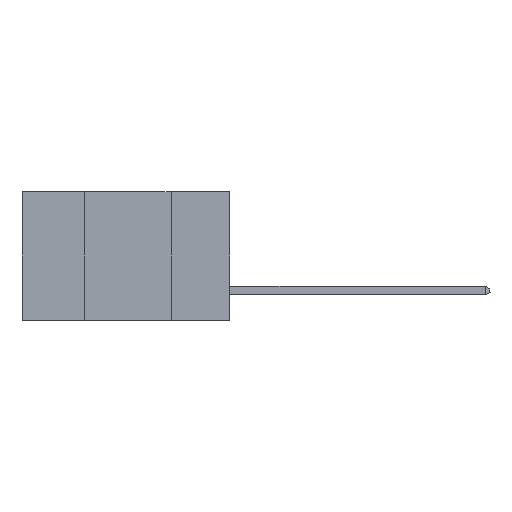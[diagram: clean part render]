
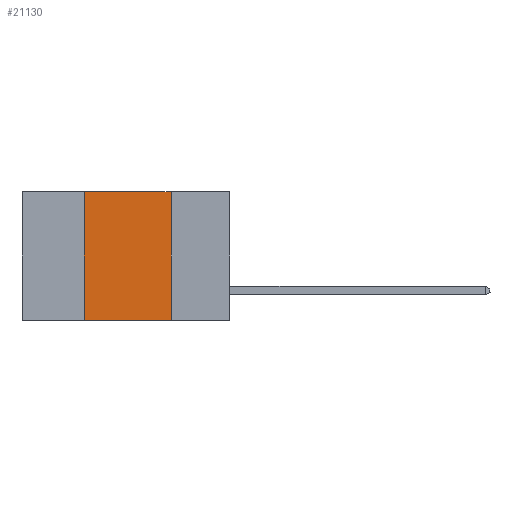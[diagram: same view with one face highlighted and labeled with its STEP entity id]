
A CAD part, left-side view. The second image highlights one B-rep face of the part: STEP entity #21130.
In plain terms, the highlighted planar face has unit normal (-1, 0, 0).
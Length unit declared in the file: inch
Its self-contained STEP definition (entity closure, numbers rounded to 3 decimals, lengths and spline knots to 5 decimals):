
#48 = VERTEX_POINT ( 'NONE', #13141 ) ;
#565 = AXIS2_PLACEMENT_3D ( 'NONE', #20425, #24360, #592 ) ;
#592 = DIRECTION ( 'NONE',  ( 0., 0., -1. ) ) ;
#999 = CARTESIAN_POINT ( 'NONE',  ( 0., 0.42, 0. ) ) ;
#2029 = CARTESIAN_POINT ( 'NONE',  ( 0., 0.17, 0. ) ) ;
#2533 = VECTOR ( 'NONE', #8367, 39.37008 ) ;
#2680 = LINE ( 'NONE', #2029, #4232 ) ;
#2936 = ORIENTED_EDGE ( 'NONE', *, *, #7417, .F. ) ;
#3511 = VECTOR ( 'NONE', #10953, 39.37008 ) ;
#3671 = ORIENTED_EDGE ( 'NONE', *, *, #24396, .F. ) ;
#3968 = EDGE_CURVE ( 'NONE', #14543, #48, #8791, .T. ) ;
#3976 = DIRECTION ( 'NONE',  ( 0., 0., -1. ) ) ;
#4232 = VECTOR ( 'NONE', #3976, 39.37008 ) ;
#4890 = ORIENTED_EDGE ( 'NONE', *, *, #3968, .F. ) ;
#5565 = FACE_OUTER_BOUND ( 'NONE', #9289, .T. ) ;
#7417 = EDGE_CURVE ( 'NONE', #48, #22694, #2680, .T. ) ;
#8367 = DIRECTION ( 'NONE',  ( 0., -1., 0. ) ) ;
#8791 = LINE ( 'NONE', #16941, #3511 ) ;
#9289 = EDGE_LOOP ( 'NONE', ( #2936, #4890, #3671, #21521 ) ) ;
#9727 = LINE ( 'NONE', #12284, #2533 ) ;
#9985 = CARTESIAN_POINT ( 'NONE',  ( 0., 0.42, 0. ) ) ;
#10711 = DIRECTION ( 'NONE',  ( 0., 0., 1. ) ) ;
#10953 = DIRECTION ( 'NONE',  ( 0., -1., 0. ) ) ;
#12284 = CARTESIAN_POINT ( 'NONE',  ( 0., 0.6, -0.37 ) ) ;
#13141 = CARTESIAN_POINT ( 'NONE',  ( 0., 0.17, 0. ) ) ;
#14543 = VERTEX_POINT ( 'NONE', #9985 ) ;
#16307 = CARTESIAN_POINT ( 'NONE',  ( 0., 0.17, -0.37 ) ) ;
#16941 = CARTESIAN_POINT ( 'NONE',  ( 0., 0.6, 0. ) ) ;
#17818 = LINE ( 'NONE', #999, #23947 ) ;
#19235 = EDGE_CURVE ( 'NONE', #24917, #22694, #9727, .T. ) ;
#20425 = CARTESIAN_POINT ( 'NONE',  ( 0., 0.6, 0. ) ) ;
#20536 = CARTESIAN_POINT ( 'NONE',  ( 0., 0.42, -0.37 ) ) ;
#21130 = ADVANCED_FACE ( 'NONE', ( #5565 ), #22457, .F. ) ;
#21521 = ORIENTED_EDGE ( 'NONE', *, *, #19235, .T. ) ;
#22457 = PLANE ( 'NONE',  #565 ) ;
#22694 = VERTEX_POINT ( 'NONE', #16307 ) ;
#23947 = VECTOR ( 'NONE', #10711, 39.37008 ) ;
#24360 = DIRECTION ( 'NONE',  ( 1., 0., 0. ) ) ;
#24396 = EDGE_CURVE ( 'NONE', #24917, #14543, #17818, .T. ) ;
#24917 = VERTEX_POINT ( 'NONE', #20536 ) ;
